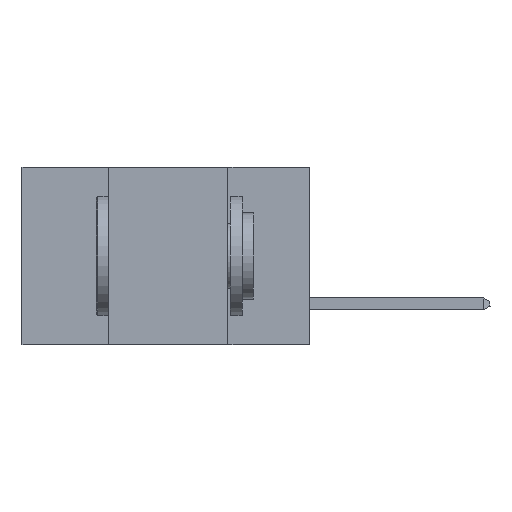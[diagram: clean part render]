
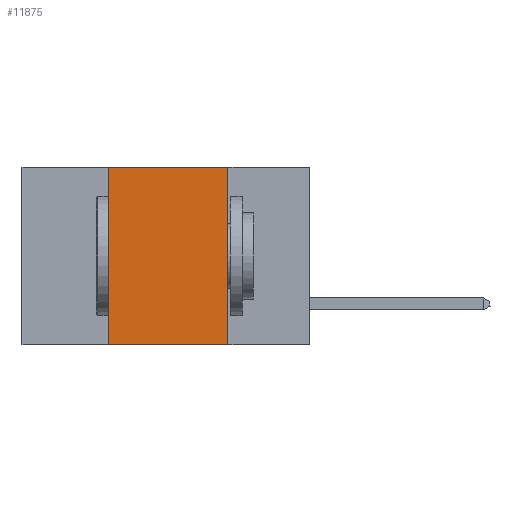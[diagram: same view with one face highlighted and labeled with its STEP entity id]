
A CAD part, left-side view. The second image highlights one B-rep face of the part: STEP entity #11875.
In plain terms, the highlighted planar face has unit normal (-1, 0, 0).
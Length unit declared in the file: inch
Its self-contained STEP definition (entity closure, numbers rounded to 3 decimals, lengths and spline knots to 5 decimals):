
#103 = LINE ( 'NONE', #8796, #16486 ) ;
#503 = EDGE_LOOP ( 'NONE', ( #6797, #14496, #2957, #3584 ) ) ;
#1021 = DIRECTION ( 'NONE',  ( 0., -1., 0. ) ) ;
#1071 = EDGE_CURVE ( 'NONE', #16620, #13633, #13441, .T. ) ;
#1841 = LINE ( 'NONE', #15488, #8154 ) ;
#2395 = EDGE_CURVE ( 'NONE', #4784, #3491, #103, .T. ) ;
#2957 = ORIENTED_EDGE ( 'NONE', *, *, #7064, .F. ) ;
#3491 = VERTEX_POINT ( 'NONE', #14801 ) ;
#3584 = ORIENTED_EDGE ( 'NONE', *, *, #2395, .T. ) ;
#4109 = CARTESIAN_POINT ( 'NONE',  ( 0., 0.42, 0. ) ) ;
#4784 = VERTEX_POINT ( 'NONE', #8339 ) ;
#4865 = CARTESIAN_POINT ( 'NONE',  ( 0., 0.6, 0. ) ) ;
#4913 = DIRECTION ( 'NONE',  ( 1., 0., 0. ) ) ;
#6797 = ORIENTED_EDGE ( 'NONE', *, *, #8928, .F. ) ;
#6925 = DIRECTION ( 'NONE',  ( 0., -1., 0. ) ) ;
#7064 = EDGE_CURVE ( 'NONE', #4784, #16620, #10896, .T. ) ;
#7112 = CARTESIAN_POINT ( 'NONE',  ( 0., 0.17, 0. ) ) ;
#7599 = PLANE ( 'NONE',  #14479 ) ;
#8154 = VECTOR ( 'NONE', #14389, 39.37008 ) ;
#8339 = CARTESIAN_POINT ( 'NONE',  ( 0., 0.42, -0.37 ) ) ;
#8603 = CARTESIAN_POINT ( 'NONE',  ( 0., 0.42, 0. ) ) ;
#8796 = CARTESIAN_POINT ( 'NONE',  ( 0., 0.6, -0.37 ) ) ;
#8928 = EDGE_CURVE ( 'NONE', #13633, #3491, #1841, .T. ) ;
#9953 = VECTOR ( 'NONE', #6925, 39.37008 ) ;
#10209 = DIRECTION ( 'NONE',  ( 0., 0., -1. ) ) ;
#10549 = FACE_OUTER_BOUND ( 'NONE', #503, .T. ) ;
#10896 = LINE ( 'NONE', #8603, #14785 ) ;
#11875 = ADVANCED_FACE ( 'NONE', ( #10549 ), #7599, .F. ) ;
#13441 = LINE ( 'NONE', #14836, #9953 ) ;
#13633 = VERTEX_POINT ( 'NONE', #7112 ) ;
#14389 = DIRECTION ( 'NONE',  ( 0., 0., -1. ) ) ;
#14479 = AXIS2_PLACEMENT_3D ( 'NONE', #4865, #4913, #10209 ) ;
#14496 = ORIENTED_EDGE ( 'NONE', *, *, #1071, .F. ) ;
#14785 = VECTOR ( 'NONE', #16599, 39.37008 ) ;
#14801 = CARTESIAN_POINT ( 'NONE',  ( 0., 0.17, -0.37 ) ) ;
#14836 = CARTESIAN_POINT ( 'NONE',  ( 0., 0.6, 0. ) ) ;
#15488 = CARTESIAN_POINT ( 'NONE',  ( 0., 0.17, 0. ) ) ;
#16486 = VECTOR ( 'NONE', #1021, 39.37008 ) ;
#16599 = DIRECTION ( 'NONE',  ( 0., 0., 1. ) ) ;
#16620 = VERTEX_POINT ( 'NONE', #4109 ) ;
